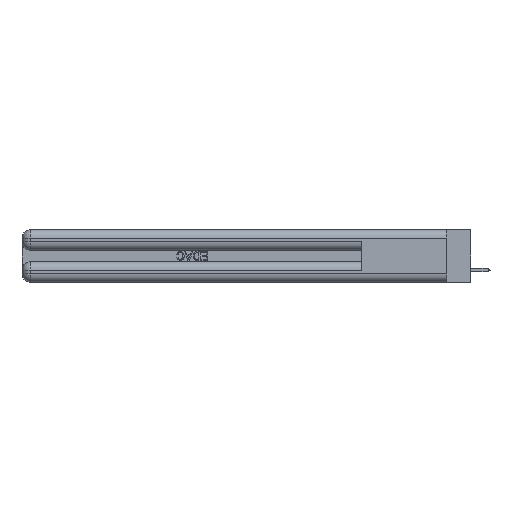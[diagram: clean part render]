
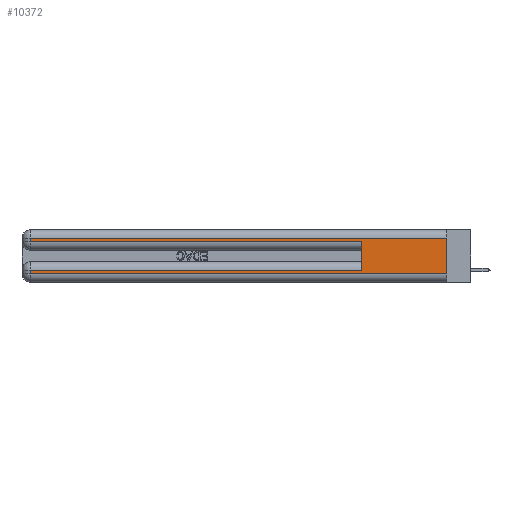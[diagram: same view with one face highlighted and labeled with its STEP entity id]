
A CAD part, left-side view. The second image highlights one B-rep face of the part: STEP entity #10372.
In plain terms, the highlighted planar face has unit normal (-1, 0, 0).
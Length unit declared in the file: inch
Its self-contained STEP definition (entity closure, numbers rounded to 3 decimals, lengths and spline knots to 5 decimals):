
#330 = EDGE_CURVE ( 'NONE', #27672, #12098, #36746, .T. ) ;
#2521 = EDGE_CURVE ( 'NONE', #16641, #11424, #37902, .T. ) ;
#3673 = DIRECTION ( 'NONE',  ( 0., -1., 0. ) ) ;
#4196 = LINE ( 'NONE', #38775, #28507 ) ;
#4522 = DIRECTION ( 'NONE',  ( 0., 0., -1. ) ) ;
#4670 = CARTESIAN_POINT ( 'NONE',  ( 0., 0., 0.06 ) ) ;
#5223 = ORIENTED_EDGE ( 'NONE', *, *, #26932, .T. ) ;
#5915 = EDGE_CURVE ( 'NONE', #11424, #12323, #32873, .T. ) ;
#5931 = VECTOR ( 'NONE', #6429, 39.37008 ) ;
#6429 = DIRECTION ( 'NONE',  ( 0., 1., 0. ) ) ;
#6761 = ORIENTED_EDGE ( 'NONE', *, *, #2521, .T. ) ;
#8476 = VECTOR ( 'NONE', #13915, 39.37008 ) ;
#8871 = FACE_OUTER_BOUND ( 'NONE', #38847, .T. ) ;
#9174 = ORIENTED_EDGE ( 'NONE', *, *, #9554, .T. ) ;
#9554 = EDGE_CURVE ( 'NONE', #20191, #27672, #4196, .T. ) ;
#10103 = CARTESIAN_POINT ( 'NONE',  ( 0., 0., 0.37 ) ) ;
#10372 = ADVANCED_FACE ( 'NONE', ( #8871 ), #25177, .F. ) ;
#10893 = VERTEX_POINT ( 'NONE', #13089 ) ;
#11424 = VERTEX_POINT ( 'NONE', #19648 ) ;
#11861 = ORIENTED_EDGE ( 'NONE', *, *, #14868, .F. ) ;
#12098 = VERTEX_POINT ( 'NONE', #26865 ) ;
#12323 = VERTEX_POINT ( 'NONE', #27032 ) ;
#12889 = VECTOR ( 'NONE', #38826, 39.37008 ) ;
#13089 = CARTESIAN_POINT ( 'NONE',  ( 0., 0., 0.06 ) ) ;
#13915 = DIRECTION ( 'NONE',  ( 0., 1., 0. ) ) ;
#14333 = DIRECTION ( 'NONE',  ( 0., 0., -1. ) ) ;
#14751 = LINE ( 'NONE', #34789, #8476 ) ;
#14868 = EDGE_CURVE ( 'NONE', #26977, #10893, #24338, .T. ) ;
#16343 = VECTOR ( 'NONE', #31410, 39.37008 ) ;
#16641 = VERTEX_POINT ( 'NONE', #33761 ) ;
#17520 = AXIS2_PLACEMENT_3D ( 'NONE', #10103, #22668, #37571 ) ;
#19634 = VECTOR ( 'NONE', #3673, 39.37008 ) ;
#19648 = CARTESIAN_POINT ( 'NONE',  ( 0., 2.94, 0.085 ) ) ;
#20191 = VERTEX_POINT ( 'NONE', #33090 ) ;
#20771 = CARTESIAN_POINT ( 'NONE',  ( 0., 2.94, 0.37 ) ) ;
#21385 = CARTESIAN_POINT ( 'NONE',  ( 0., 0., 0.31 ) ) ;
#22668 = DIRECTION ( 'NONE',  ( 1., 0., 0. ) ) ;
#23536 = ORIENTED_EDGE ( 'NONE', *, *, #330, .T. ) ;
#24338 = LINE ( 'NONE', #39086, #12889 ) ;
#25177 = PLANE ( 'NONE',  #17520 ) ;
#26576 = EDGE_CURVE ( 'NONE', #16641, #12098, #29659, .T. ) ;
#26865 = CARTESIAN_POINT ( 'NONE',  ( 0., 0.6, 0.285 ) ) ;
#26932 = EDGE_CURVE ( 'NONE', #12323, #10893, #27594, .T. ) ;
#26977 = VERTEX_POINT ( 'NONE', #21385 ) ;
#27032 = CARTESIAN_POINT ( 'NONE',  ( 0., 2.94, 0.06 ) ) ;
#27594 = LINE ( 'NONE', #4670, #35224 ) ;
#27672 = VERTEX_POINT ( 'NONE', #30572 ) ;
#28507 = VECTOR ( 'NONE', #14333, 39.37008 ) ;
#29588 = ORIENTED_EDGE ( 'NONE', *, *, #26576, .F. ) ;
#29659 = LINE ( 'NONE', #31120, #16343 ) ;
#29996 = VECTOR ( 'NONE', #4522, 39.37008 ) ;
#30572 = CARTESIAN_POINT ( 'NONE',  ( 0., 2.94, 0.285 ) ) ;
#30678 = CARTESIAN_POINT ( 'NONE',  ( 0., 0., 0.085 ) ) ;
#31120 = CARTESIAN_POINT ( 'NONE',  ( 0., 0.6, 0.145 ) ) ;
#31410 = DIRECTION ( 'NONE',  ( 0., 0., 1. ) ) ;
#32873 = LINE ( 'NONE', #20771, #29996 ) ;
#33090 = CARTESIAN_POINT ( 'NONE',  ( 0., 2.94, 0.31 ) ) ;
#33676 = EDGE_CURVE ( 'NONE', #26977, #20191, #14751, .T. ) ;
#33761 = CARTESIAN_POINT ( 'NONE',  ( 0., 0.6, 0.085 ) ) ;
#34783 = ORIENTED_EDGE ( 'NONE', *, *, #33676, .T. ) ;
#34789 = CARTESIAN_POINT ( 'NONE',  ( 0., 0., 0.31 ) ) ;
#35224 = VECTOR ( 'NONE', #38598, 39.37008 ) ;
#36702 = CARTESIAN_POINT ( 'NONE',  ( 0., 0., 0.285 ) ) ;
#36746 = LINE ( 'NONE', #36702, #19634 ) ;
#37571 = DIRECTION ( 'NONE',  ( 0., 0., -1. ) ) ;
#37902 = LINE ( 'NONE', #30678, #5931 ) ;
#38340 = ORIENTED_EDGE ( 'NONE', *, *, #5915, .T. ) ;
#38598 = DIRECTION ( 'NONE',  ( 0., -1., 0. ) ) ;
#38775 = CARTESIAN_POINT ( 'NONE',  ( 0., 2.94, 0.37 ) ) ;
#38826 = DIRECTION ( 'NONE',  ( 0., 0., -1. ) ) ;
#38847 = EDGE_LOOP ( 'NONE', ( #11861, #34783, #9174, #23536, #29588, #6761, #38340, #5223 ) ) ;
#39086 = CARTESIAN_POINT ( 'NONE',  ( 0., 0., 0.37 ) ) ;
